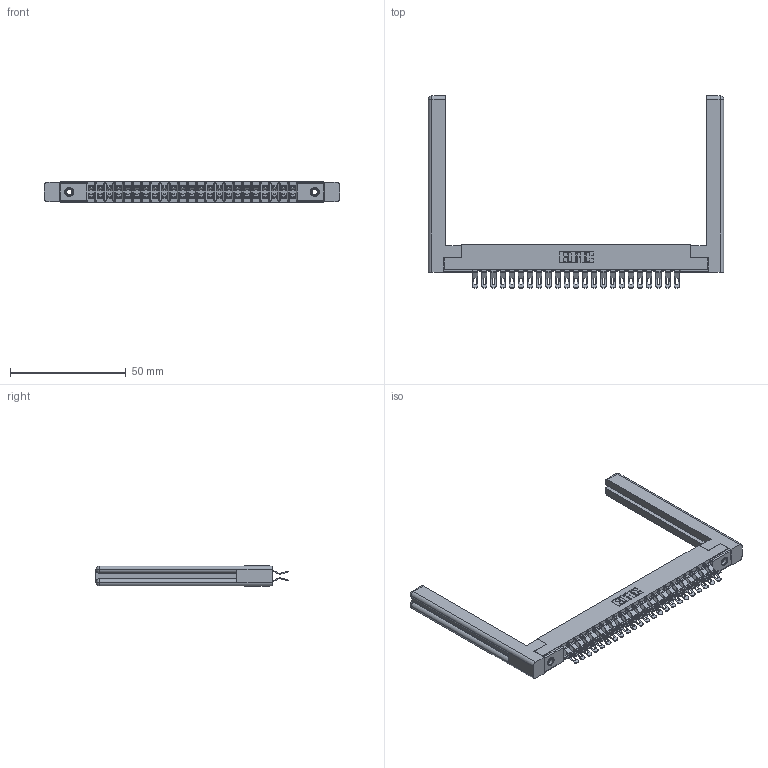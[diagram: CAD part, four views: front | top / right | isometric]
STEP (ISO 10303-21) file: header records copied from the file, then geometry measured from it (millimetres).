
FILE_DESCRIPTION (( 'STEP AP203' ), '1' );
FILE_NAME ('357-046-555-258.STEP', '2019-09-18T08:47:29', ( '' ), ( '' ), 'SwSTEP 2.0', 'SolidWorks 2016', '' );
FILE_SCHEMA (( 'CONFIG_CONTROL_DESIGN' ));
Length unit declared in the file: inch
Products named in the file (5): 357-046-555-258; 307-220-058; 345-250-001_345-250-001-102; 307 Part_.156 Dia Mounting Holes; 307-290-001_555
Assembly tree (51 placements, depth 2):
  357-046-555-258
    307 Part_.156 Dia Mounting Holes
    307-290-001_555  x46
    307-220-058  x2
    345-250-001_345-250-001-102  x2
Bounding box: 127.76 x 83.06 x 8.71 mm (x, y, z)
Volume: 16180.6 mm3; surface area: 20901 mm2
Topology: 51 solids, 51 shells, 3090 faces, 9003 edges, 5862 vertices
Faces by surface type: plane 1718, cylinder 1300, sphere 48, torus 12, cone 12
Entity records: 25966 total; most frequent: CARTESIAN_POINT 4278, ORIENTED_EDGE 4182, DIRECTION 4163, EDGE_CURVE 2091, VECTOR 1581, LINE 1581, VERTEX_POINT 1352, AXIS2_PLACEMENT_3D 1291
